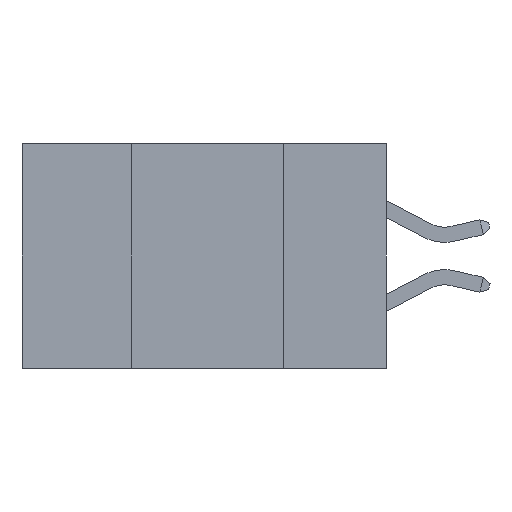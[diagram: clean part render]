
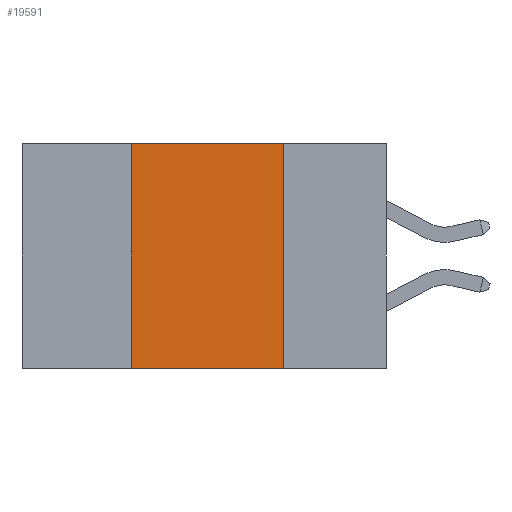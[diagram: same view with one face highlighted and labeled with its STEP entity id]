
A CAD part, left-side view. The second image highlights one B-rep face of the part: STEP entity #19591.
In plain terms, the highlighted planar face has unit normal (-1, 0, 0).
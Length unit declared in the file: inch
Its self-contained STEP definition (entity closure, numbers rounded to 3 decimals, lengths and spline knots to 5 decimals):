
#9 = CARTESIAN_POINT ( 'NONE',  ( 0., 0.17, -0.37 ) ) ;
#58 = DIRECTION ( 'NONE',  ( 0., -1., 0. ) ) ;
#1284 = DIRECTION ( 'NONE',  ( 1., 0., 0. ) ) ;
#1616 = VERTEX_POINT ( 'NONE', #16630 ) ;
#3980 = LINE ( 'NONE', #17183, #13466 ) ;
#4626 = ORIENTED_EDGE ( 'NONE', *, *, #22366, .T. ) ;
#6304 = VECTOR ( 'NONE', #13426, 39.37008 ) ;
#7603 = VERTEX_POINT ( 'NONE', #22028 ) ;
#9765 = DIRECTION ( 'NONE',  ( 0., -1., 0. ) ) ;
#10367 = EDGE_LOOP ( 'NONE', ( #19896, #13516, #19020, #4626 ) ) ;
#10531 = VERTEX_POINT ( 'NONE', #11259 ) ;
#11259 = CARTESIAN_POINT ( 'NONE',  ( 0., 0.42, 0. ) ) ;
#11928 = DIRECTION ( 'NONE',  ( 0., 0., 1. ) ) ;
#12011 = EDGE_CURVE ( 'NONE', #10531, #7603, #3980, .T. ) ;
#12669 = CARTESIAN_POINT ( 'NONE',  ( 0., 0.6, 0. ) ) ;
#13201 = LINE ( 'NONE', #13801, #22472 ) ;
#13273 = EDGE_CURVE ( 'NONE', #7603, #1616, #24436, .T. ) ;
#13426 = DIRECTION ( 'NONE',  ( 0., 0., -1. ) ) ;
#13466 = VECTOR ( 'NONE', #9765, 39.37008 ) ;
#13516 = ORIENTED_EDGE ( 'NONE', *, *, #12011, .F. ) ;
#13758 = LINE ( 'NONE', #22701, #23028 ) ;
#13801 = CARTESIAN_POINT ( 'NONE',  ( 0., 0.42, -0.37 ) ) ;
#14521 = AXIS2_PLACEMENT_3D ( 'NONE', #12669, #1284, #14624 ) ;
#14624 = DIRECTION ( 'NONE',  ( 0., 0., -1. ) ) ;
#15567 = VERTEX_POINT ( 'NONE', #20359 ) ;
#16630 = CARTESIAN_POINT ( 'NONE',  ( 0., 0.17, -0.37 ) ) ;
#17183 = CARTESIAN_POINT ( 'NONE',  ( 0., 0.6, 0. ) ) ;
#19020 = ORIENTED_EDGE ( 'NONE', *, *, #21962, .F. ) ;
#19591 = ADVANCED_FACE ( 'NONE', ( #22929 ), #23868, .F. ) ;
#19896 = ORIENTED_EDGE ( 'NONE', *, *, #13273, .F. ) ;
#20359 = CARTESIAN_POINT ( 'NONE',  ( 0., 0.42, -0.37 ) ) ;
#21962 = EDGE_CURVE ( 'NONE', #15567, #10531, #13201, .T. ) ;
#22028 = CARTESIAN_POINT ( 'NONE',  ( 0., 0.17, 0. ) ) ;
#22366 = EDGE_CURVE ( 'NONE', #15567, #1616, #13758, .T. ) ;
#22472 = VECTOR ( 'NONE', #11928, 39.37008 ) ;
#22701 = CARTESIAN_POINT ( 'NONE',  ( 0., 0.6, -0.37 ) ) ;
#22929 = FACE_OUTER_BOUND ( 'NONE', #10367, .T. ) ;
#23028 = VECTOR ( 'NONE', #58, 39.37008 ) ;
#23868 = PLANE ( 'NONE',  #14521 ) ;
#24436 = LINE ( 'NONE', #9, #6304 ) ;
